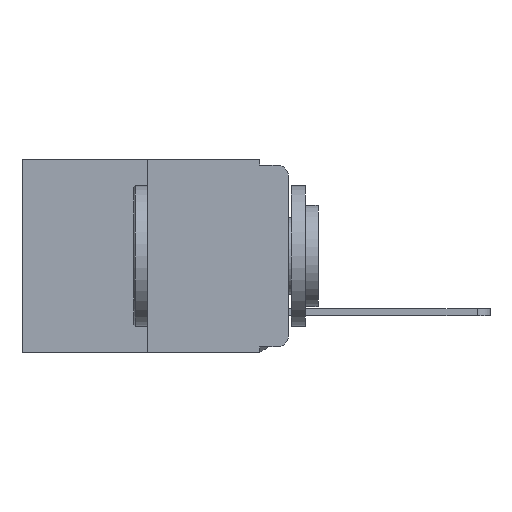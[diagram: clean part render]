
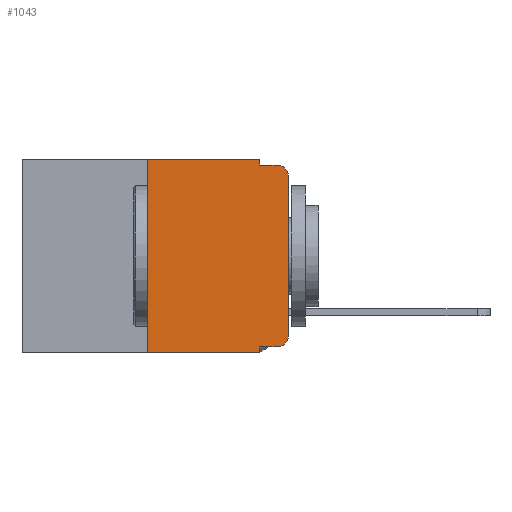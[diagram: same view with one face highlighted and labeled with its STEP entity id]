
A CAD part, left-side view. The second image highlights one B-rep face of the part: STEP entity #1043.
In plain terms, the highlighted planar face has unit normal (-1, 0, 0).
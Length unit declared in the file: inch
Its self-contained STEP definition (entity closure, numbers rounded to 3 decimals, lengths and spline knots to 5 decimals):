
#2 = LINE ( 'NONE', #1977, #16148 ) ;
#10 = VERTEX_POINT ( 'NONE', #12371 ) ;
#25 = DIRECTION ( 'NONE',  ( 0., -1., 0. ) ) ;
#454 = CARTESIAN_POINT ( 'NONE',  ( 0., 0.051, -0.01 ) ) ;
#477 = VERTEX_POINT ( 'NONE', #2236 ) ;
#686 = VERTEX_POINT ( 'NONE', #1973 ) ;
#1043 = ADVANCED_FACE ( 'NONE', ( #15841 ), #6416, .F. ) ;
#1285 = CARTESIAN_POINT ( 'NONE',  ( 0., 0.473, 0. ) ) ;
#1384 = CARTESIAN_POINT ( 'NONE',  ( 0., 0.473, -0.343 ) ) ;
#1456 = VERTEX_POINT ( 'NONE', #3365 ) ;
#1904 = EDGE_CURVE ( 'NONE', #3762, #3096, #17200, .T. ) ;
#1973 = CARTESIAN_POINT ( 'NONE',  ( 0., 0.051, -0.333 ) ) ;
#1977 = CARTESIAN_POINT ( 'NONE',  ( 0., 0.051, -0.333 ) ) ;
#2002 = DIRECTION ( 'NONE',  ( 0., -1., 0. ) ) ;
#2041 = EDGE_CURVE ( 'NONE', #686, #3096, #18814, .T. ) ;
#2059 = DIRECTION ( 'NONE',  ( 0., -1., 0. ) ) ;
#2236 = CARTESIAN_POINT ( 'NONE',  ( 0., 0.25, 0. ) ) ;
#2944 = CIRCLE ( 'NONE', #6540, 0.02 ) ;
#3049 = EDGE_LOOP ( 'NONE', ( #11116, #15023, #11592, #15946, #4290, #8509, #4773, #8987, #13438, #17343 ) ) ;
#3058 = VECTOR ( 'NONE', #12406, 39.37008 ) ;
#3096 = VERTEX_POINT ( 'NONE', #3750 ) ;
#3288 = DIRECTION ( 'NONE',  ( -1., 0., 0. ) ) ;
#3365 = CARTESIAN_POINT ( 'NONE',  ( 0., 0., -0.03 ) ) ;
#3416 = DIRECTION ( 'NONE',  ( -1., 0., 0. ) ) ;
#3418 = CARTESIAN_POINT ( 'NONE',  ( 0., 0.25, 0. ) ) ;
#3750 = CARTESIAN_POINT ( 'NONE',  ( 0., 0.051, -0.343 ) ) ;
#3762 = VERTEX_POINT ( 'NONE', #9426 ) ;
#4290 = ORIENTED_EDGE ( 'NONE', *, *, #18217, .F. ) ;
#4489 = DIRECTION ( 'NONE',  ( 0., 0., 1. ) ) ;
#4714 = LINE ( 'NONE', #12486, #8437 ) ;
#4773 = ORIENTED_EDGE ( 'NONE', *, *, #1904, .T. ) ;
#5210 = LINE ( 'NONE', #13699, #13390 ) ;
#6291 = CARTESIAN_POINT ( 'NONE',  ( 0., 0.02, -0.01 ) ) ;
#6387 = AXIS2_PLACEMENT_3D ( 'NONE', #12712, #3416, #14181 ) ;
#6416 = PLANE ( 'NONE',  #8390 ) ;
#6434 = CARTESIAN_POINT ( 'NONE',  ( 0., 0.473, 0. ) ) ;
#6540 = AXIS2_PLACEMENT_3D ( 'NONE', #12601, #3288, #14062 ) ;
#7285 = VERTEX_POINT ( 'NONE', #454 ) ;
#8390 = AXIS2_PLACEMENT_3D ( 'NONE', #6434, #10119, #10114 ) ;
#8437 = VECTOR ( 'NONE', #19768, 39.37008 ) ;
#8508 = EDGE_CURVE ( 'NONE', #3762, #477, #12742, .T. ) ;
#8509 = ORIENTED_EDGE ( 'NONE', *, *, #8508, .F. ) ;
#8987 = ORIENTED_EDGE ( 'NONE', *, *, #2041, .F. ) ;
#9221 = VECTOR ( 'NONE', #14182, 39.37008 ) ;
#9426 = CARTESIAN_POINT ( 'NONE',  ( 0., 0.25, -0.343 ) ) ;
#9541 = EDGE_CURVE ( 'NONE', #10, #7285, #4714, .T. ) ;
#10023 = VECTOR ( 'NONE', #25, 39.37008 ) ;
#10114 = DIRECTION ( 'NONE',  ( 0., 0., -1. ) ) ;
#10119 = DIRECTION ( 'NONE',  ( 1., 0., 0. ) ) ;
#11116 = ORIENTED_EDGE ( 'NONE', *, *, #15479, .T. ) ;
#11592 = ORIENTED_EDGE ( 'NONE', *, *, #12561, .F. ) ;
#11832 = CARTESIAN_POINT ( 'NONE',  ( 0., 0.02, -0.333 ) ) ;
#12371 = CARTESIAN_POINT ( 'NONE',  ( 0., 0.051, 0. ) ) ;
#12406 = DIRECTION ( 'NONE',  ( 0., -1., 0. ) ) ;
#12486 = CARTESIAN_POINT ( 'NONE',  ( 0., 0.051, 0. ) ) ;
#12561 = EDGE_CURVE ( 'NONE', #7285, #14421, #17865, .T. ) ;
#12601 = CARTESIAN_POINT ( 'NONE',  ( 0., 0.02, -0.313 ) ) ;
#12712 = CARTESIAN_POINT ( 'NONE',  ( 0., 0.02, -0.03 ) ) ;
#12742 = LINE ( 'NONE', #3418, #9221 ) ;
#13321 = VECTOR ( 'NONE', #2002, 39.37008 ) ;
#13390 = VECTOR ( 'NONE', #4489, 39.37008 ) ;
#13438 = ORIENTED_EDGE ( 'NONE', *, *, #19782, .T. ) ;
#13699 = CARTESIAN_POINT ( 'NONE',  ( 0., 0., 0. ) ) ;
#14062 = DIRECTION ( 'NONE',  ( 0., 0., -1. ) ) ;
#14181 = DIRECTION ( 'NONE',  ( 0., 0., -1. ) ) ;
#14182 = DIRECTION ( 'NONE',  ( 0., 0., 1. ) ) ;
#14292 = VERTEX_POINT ( 'NONE', #18568 ) ;
#14421 = VERTEX_POINT ( 'NONE', #6291 ) ;
#14524 = EDGE_CURVE ( 'NONE', #1456, #14421, #16632, .T. ) ;
#14878 = CARTESIAN_POINT ( 'NONE',  ( 0., 0.051, 0. ) ) ;
#14886 = VECTOR ( 'NONE', #15002, 39.37008 ) ;
#15002 = DIRECTION ( 'NONE',  ( 0., 0., -1. ) ) ;
#15023 = ORIENTED_EDGE ( 'NONE', *, *, #14524, .T. ) ;
#15287 = LINE ( 'NONE', #1285, #3058 ) ;
#15479 = EDGE_CURVE ( 'NONE', #14292, #1456, #5210, .T. ) ;
#15841 = FACE_OUTER_BOUND ( 'NONE', #3049, .T. ) ;
#15855 = EDGE_CURVE ( 'NONE', #17998, #14292, #2944, .T. ) ;
#15946 = ORIENTED_EDGE ( 'NONE', *, *, #9541, .F. ) ;
#16148 = VECTOR ( 'NONE', #2059, 39.37008 ) ;
#16632 = CIRCLE ( 'NONE', #6387, 0.02 ) ;
#17200 = LINE ( 'NONE', #1384, #13321 ) ;
#17343 = ORIENTED_EDGE ( 'NONE', *, *, #15855, .T. ) ;
#17865 = LINE ( 'NONE', #18594, #10023 ) ;
#17998 = VERTEX_POINT ( 'NONE', #11832 ) ;
#18217 = EDGE_CURVE ( 'NONE', #477, #10, #15287, .T. ) ;
#18568 = CARTESIAN_POINT ( 'NONE',  ( 0., 0., -0.313 ) ) ;
#18594 = CARTESIAN_POINT ( 'NONE',  ( 0., 0.051, -0.01 ) ) ;
#18814 = LINE ( 'NONE', #14878, #14886 ) ;
#19768 = DIRECTION ( 'NONE',  ( 0., 0., -1. ) ) ;
#19782 = EDGE_CURVE ( 'NONE', #686, #17998, #2, .T. ) ;
